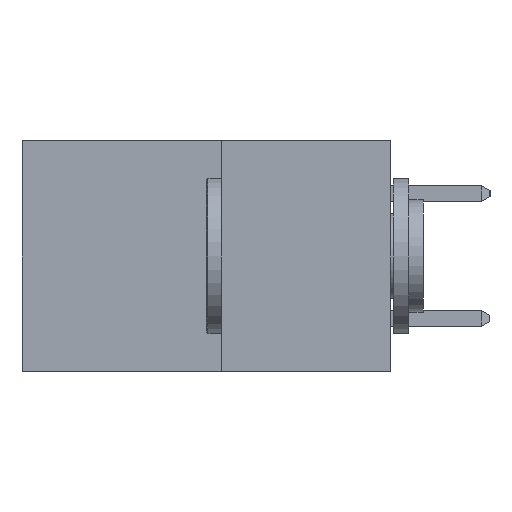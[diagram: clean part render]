
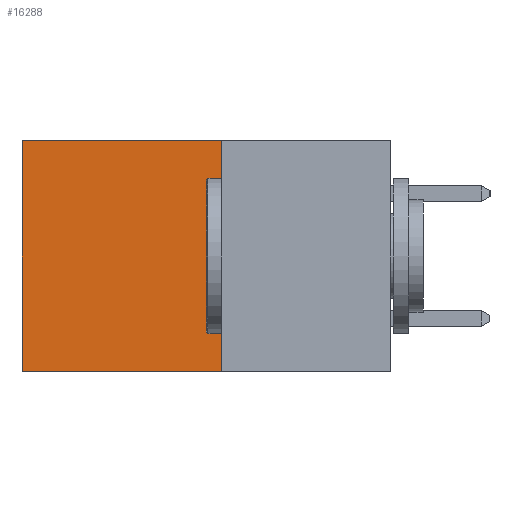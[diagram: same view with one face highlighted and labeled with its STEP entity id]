
A CAD part, left-side view. The second image highlights one B-rep face of the part: STEP entity #16288.
In plain terms, the highlighted planar face has unit normal (-1, 0, 0).
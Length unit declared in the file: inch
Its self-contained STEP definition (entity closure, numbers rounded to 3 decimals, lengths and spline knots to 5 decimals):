
#713 = FACE_OUTER_BOUND ( 'NONE', #1728, .T. ) ;
#848 = DIRECTION ( 'NONE',  ( 1., 0., 0. ) ) ;
#1161 = VECTOR ( 'NONE', #13673, 39.37008 ) ;
#1728 = EDGE_LOOP ( 'NONE', ( #9588, #20015, #3356, #19671 ) ) ;
#2123 = CARTESIAN_POINT ( 'NONE',  ( 0.277, 0.27, -0.37 ) ) ;
#2314 = VECTOR ( 'NONE', #11573, 39.37008 ) ;
#2494 = VERTEX_POINT ( 'NONE', #18603 ) ;
#3282 = LINE ( 'NONE', #9494, #19841 ) ;
#3356 = ORIENTED_EDGE ( 'NONE', *, *, #6816, .F. ) ;
#4043 = EDGE_CURVE ( 'NONE', #12632, #6695, #9941, .T. ) ;
#4246 = CARTESIAN_POINT ( 'NONE',  ( 0.277, 0.27, -0.37 ) ) ;
#4683 = EDGE_CURVE ( 'NONE', #20224, #6695, #12287, .T. ) ;
#6695 = VERTEX_POINT ( 'NONE', #18019 ) ;
#6816 = EDGE_CURVE ( 'NONE', #2494, #20224, #3282, .T. ) ;
#9021 = DIRECTION ( 'NONE',  ( 0., 0., -1. ) ) ;
#9494 = CARTESIAN_POINT ( 'NONE',  ( 0.277, 0.27, -0.37 ) ) ;
#9588 = ORIENTED_EDGE ( 'NONE', *, *, #4043, .T. ) ;
#9941 = LINE ( 'NONE', #17876, #2314 ) ;
#10674 = AXIS2_PLACEMENT_3D ( 'NONE', #4246, #848, #12864 ) ;
#11225 = PLANE ( 'NONE',  #10674 ) ;
#11237 = VECTOR ( 'NONE', #16953, 39.37008 ) ;
#11411 = CARTESIAN_POINT ( 'NONE',  ( 0.277, 0.59, 0. ) ) ;
#11573 = DIRECTION ( 'NONE',  ( 0., 0., -1. ) ) ;
#11743 = EDGE_CURVE ( 'NONE', #2494, #12632, #14716, .T. ) ;
#12287 = LINE ( 'NONE', #16837, #11237 ) ;
#12632 = VERTEX_POINT ( 'NONE', #11411 ) ;
#12864 = DIRECTION ( 'NONE',  ( 0., 0., -1. ) ) ;
#13673 = DIRECTION ( 'NONE',  ( 0., 1., 0. ) ) ;
#14716 = LINE ( 'NONE', #20011, #1161 ) ;
#16288 = ADVANCED_FACE ( 'NONE', ( #713 ), #11225, .F. ) ;
#16837 = CARTESIAN_POINT ( 'NONE',  ( 0.277, 0.27, -0.37 ) ) ;
#16953 = DIRECTION ( 'NONE',  ( 0., 1., 0. ) ) ;
#17876 = CARTESIAN_POINT ( 'NONE',  ( 0.277, 0.59, -0.37 ) ) ;
#18019 = CARTESIAN_POINT ( 'NONE',  ( 0.277, 0.59, -0.37 ) ) ;
#18603 = CARTESIAN_POINT ( 'NONE',  ( 0.277, 0.27, 0. ) ) ;
#19671 = ORIENTED_EDGE ( 'NONE', *, *, #11743, .T. ) ;
#19841 = VECTOR ( 'NONE', #9021, 39.37008 ) ;
#20011 = CARTESIAN_POINT ( 'NONE',  ( 0.277, 0.27, 0. ) ) ;
#20015 = ORIENTED_EDGE ( 'NONE', *, *, #4683, .F. ) ;
#20224 = VERTEX_POINT ( 'NONE', #2123 ) ;
